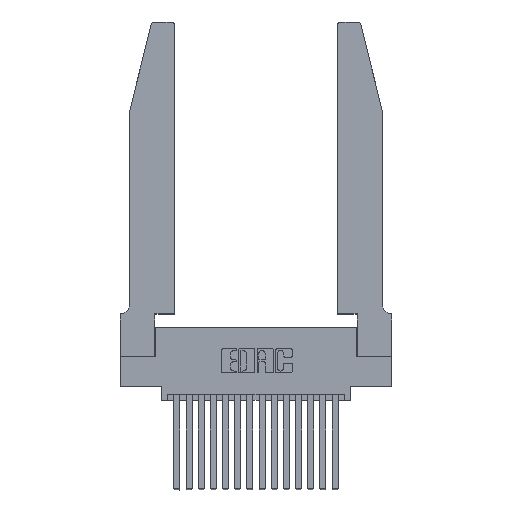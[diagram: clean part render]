
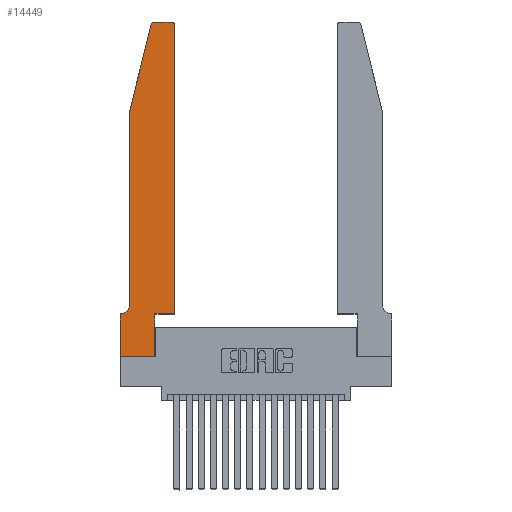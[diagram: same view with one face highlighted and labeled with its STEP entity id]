
A CAD part, top view. The second image highlights one B-rep face of the part: STEP entity #14449.
In plain terms, the highlighted planar face has unit normal (0, 0, 1).
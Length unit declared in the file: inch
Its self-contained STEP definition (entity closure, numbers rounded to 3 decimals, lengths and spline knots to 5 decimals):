
#177 = ORIENTED_EDGE ( 'NONE', *, *, #8714, .T. ) ;
#188 = AXIS2_PLACEMENT_3D ( 'NONE', #12216, #245, #10755 ) ;
#245 = DIRECTION ( 'NONE',  ( 0., 0., 1. ) ) ;
#603 = VERTEX_POINT ( 'NONE', #993 ) ;
#736 = VECTOR ( 'NONE', #13074, 39.37008 ) ;
#993 = CARTESIAN_POINT ( 'NONE',  ( 0.4505, 2.72, 0.37 ) ) ;
#1375 = AXIS2_PLACEMENT_3D ( 'NONE', #16887, #15448, #7917 ) ;
#1655 = AXIS2_PLACEMENT_3D ( 'NONE', #14983, #9304, #18419 ) ;
#1835 = EDGE_CURVE ( 'NONE', #2698, #10015, #9314, .T. ) ;
#1875 = LINE ( 'NONE', #9151, #5435 ) ;
#2230 = VERTEX_POINT ( 'NONE', #5632 ) ;
#2486 = DIRECTION ( 'NONE',  ( 0., 1., 0. ) ) ;
#2698 = VERTEX_POINT ( 'NONE', #7965 ) ;
#2702 = ORIENTED_EDGE ( 'NONE', *, *, #19317, .T. ) ;
#2794 = CARTESIAN_POINT ( 'NONE',  ( 0.0055, 0.42, 0.37 ) ) ;
#2867 = VECTOR ( 'NONE', #10861, 39.37008 ) ;
#2939 = DIRECTION ( 'NONE',  ( -0.239, -0.971, 0. ) ) ;
#3143 = CARTESIAN_POINT ( 'NONE',  ( 0.2865, 0.35, 0.37 ) ) ;
#3212 = EDGE_CURVE ( 'NONE', #603, #6087, #18404, .T. ) ;
#3765 = ORIENTED_EDGE ( 'NONE', *, *, #10191, .T. ) ;
#3843 = LINE ( 'NONE', #14655, #18168 ) ;
#3904 = ORIENTED_EDGE ( 'NONE', *, *, #5916, .T. ) ;
#4519 = LINE ( 'NONE', #13797, #14395 ) ;
#4533 = DIRECTION ( 'NONE',  ( 0., -1., 0. ) ) ;
#4868 = EDGE_CURVE ( 'NONE', #6087, #14637, #15301, .T. ) ;
#4906 = PLANE ( 'NONE',  #188 ) ;
#5160 = ORIENTED_EDGE ( 'NONE', *, *, #3212, .T. ) ;
#5254 = EDGE_CURVE ( 'NONE', #10039, #19252, #15999, .T. ) ;
#5353 = VECTOR ( 'NONE', #2939, 39.37008 ) ;
#5435 = VECTOR ( 'NONE', #12134, 39.37008 ) ;
#5632 = CARTESIAN_POINT ( 'NONE',  ( 0., 0., 0.37 ) ) ;
#5649 = EDGE_CURVE ( 'NONE', #10015, #10039, #1875, .T. ) ;
#5655 = ORIENTED_EDGE ( 'NONE', *, *, #5254, .T. ) ;
#5840 = EDGE_CURVE ( 'NONE', #2230, #12924, #9612, .T. ) ;
#5916 = EDGE_CURVE ( 'NONE', #12924, #14421, #11036, .T. ) ;
#5948 = CARTESIAN_POINT ( 'NONE',  ( 0.0755, 2., 0.37 ) ) ;
#6087 = VERTEX_POINT ( 'NONE', #14029 ) ;
#6096 = CARTESIAN_POINT ( 'NONE',  ( 0.4505, 0.35, 0.37 ) ) ;
#6678 = VECTOR ( 'NONE', #12892, 39.37008 ) ;
#7103 = ORIENTED_EDGE ( 'NONE', *, *, #1835, .T. ) ;
#7500 = ORIENTED_EDGE ( 'NONE', *, *, #4868, .T. ) ;
#7827 = FACE_OUTER_BOUND ( 'NONE', #16770, .T. ) ;
#7872 = LINE ( 'NONE', #15895, #6678 ) ;
#7917 = DIRECTION ( 'NONE',  ( 1., 0., 0. ) ) ;
#7965 = CARTESIAN_POINT ( 'NONE',  ( 0.25487, 2.72718, 0.37 ) ) ;
#8046 = CARTESIAN_POINT ( 'NONE',  ( 0.0055, 0.35, 0.37 ) ) ;
#8487 = CARTESIAN_POINT ( 'NONE',  ( 0.2865, 0., 0.37 ) ) ;
#8714 = EDGE_CURVE ( 'NONE', #19252, #11439, #7872, .T. ) ;
#8892 = DIRECTION ( 'NONE',  ( 0., 0., -1. ) ) ;
#9151 = CARTESIAN_POINT ( 'NONE',  ( 0.0755, 2., 0.37 ) ) ;
#9304 = DIRECTION ( 'NONE',  ( 0., 0., 1. ) ) ;
#9314 = LINE ( 'NONE', #11943, #5353 ) ;
#9600 = ORIENTED_EDGE ( 'NONE', *, *, #14201, .T. ) ;
#9612 = LINE ( 'NONE', #15589, #18309 ) ;
#9696 = VERTEX_POINT ( 'NONE', #13891 ) ;
#10015 = VERTEX_POINT ( 'NONE', #5948 ) ;
#10039 = VERTEX_POINT ( 'NONE', #10529 ) ;
#10191 = EDGE_CURVE ( 'NONE', #14421, #9696, #4519, .T. ) ;
#10529 = CARTESIAN_POINT ( 'NONE',  ( 0.0755, 0.42, 0.37 ) ) ;
#10755 = DIRECTION ( 'NONE',  ( 1., 0., 0. ) ) ;
#10861 = DIRECTION ( 'NONE',  ( 0., 1., 0. ) ) ;
#11036 = LINE ( 'NONE', #17312, #17366 ) ;
#11439 = VERTEX_POINT ( 'NONE', #15285 ) ;
#11865 = ORIENTED_EDGE ( 'NONE', *, *, #5649, .T. ) ;
#11943 = CARTESIAN_POINT ( 'NONE',  ( 0.0755, 2., 0.37 ) ) ;
#12134 = DIRECTION ( 'NONE',  ( 0., -1., 0. ) ) ;
#12172 = DIRECTION ( 'NONE',  ( 1., 0., 0. ) ) ;
#12216 = CARTESIAN_POINT ( 'NONE',  ( 0., 0.35, 0.37 ) ) ;
#12892 = DIRECTION ( 'NONE',  ( -1., 0., 0. ) ) ;
#12924 = VERTEX_POINT ( 'NONE', #8487 ) ;
#13074 = DIRECTION ( 'NONE',  ( -1., 0., 0. ) ) ;
#13797 = CARTESIAN_POINT ( 'NONE',  ( 0.4505, 0.35, 0.37 ) ) ;
#13891 = CARTESIAN_POINT ( 'NONE',  ( 0.4505, 0.35, 0.37 ) ) ;
#14029 = CARTESIAN_POINT ( 'NONE',  ( 0.4205, 2.75, 0.37 ) ) ;
#14201 = EDGE_CURVE ( 'NONE', #11439, #2230, #3843, .T. ) ;
#14395 = VECTOR ( 'NONE', #12172, 39.37008 ) ;
#14421 = VERTEX_POINT ( 'NONE', #3143 ) ;
#14449 = ADVANCED_FACE ( 'NONE', ( #7827 ), #4906, .T. ) ;
#14637 = VERTEX_POINT ( 'NONE', #15868 ) ;
#14655 = CARTESIAN_POINT ( 'NONE',  ( 0., 0., 0.37 ) ) ;
#14983 = CARTESIAN_POINT ( 'NONE',  ( 0.4205, 2.72, 0.37 ) ) ;
#15040 = EDGE_CURVE ( 'NONE', #9696, #603, #15531, .T. ) ;
#15237 = ORIENTED_EDGE ( 'NONE', *, *, #15040, .T. ) ;
#15285 = CARTESIAN_POINT ( 'NONE',  ( 0., 0.35, 0.37 ) ) ;
#15301 = LINE ( 'NONE', #17565, #736 ) ;
#15448 = DIRECTION ( 'NONE',  ( 0., 0., 1. ) ) ;
#15531 = LINE ( 'NONE', #6096, #2867 ) ;
#15589 = CARTESIAN_POINT ( 'NONE',  ( 0., 0., 0.37 ) ) ;
#15868 = CARTESIAN_POINT ( 'NONE',  ( 0.284, 2.75, 0.37 ) ) ;
#15895 = CARTESIAN_POINT ( 'NONE',  ( 0.0755, 0.35, 0.37 ) ) ;
#15999 = CIRCLE ( 'NONE', #16894, 0.07 ) ;
#16246 = DIRECTION ( 'NONE',  ( -1., 0., 0. ) ) ;
#16770 = EDGE_LOOP ( 'NONE', ( #7500, #2702, #7103, #11865, #5655, #177, #9600, #18312, #3904, #3765, #15237, #5160 ) ) ;
#16887 = CARTESIAN_POINT ( 'NONE',  ( 0.284, 2.72, 0.37 ) ) ;
#16894 = AXIS2_PLACEMENT_3D ( 'NONE', #2794, #8892, #16246 ) ;
#17081 = DIRECTION ( 'NONE',  ( 1., 0., 0. ) ) ;
#17312 = CARTESIAN_POINT ( 'NONE',  ( 0.2865, 0.35, 0.37 ) ) ;
#17366 = VECTOR ( 'NONE', #2486, 39.37008 ) ;
#17458 = CIRCLE ( 'NONE', #1375, 0.03 ) ;
#17565 = CARTESIAN_POINT ( 'NONE',  ( 0.2605, 2.75, 0.37 ) ) ;
#18168 = VECTOR ( 'NONE', #4533, 39.37008 ) ;
#18309 = VECTOR ( 'NONE', #17081, 39.37008 ) ;
#18312 = ORIENTED_EDGE ( 'NONE', *, *, #5840, .T. ) ;
#18404 = CIRCLE ( 'NONE', #1655, 0.03 ) ;
#18419 = DIRECTION ( 'NONE',  ( 1., 0., 0. ) ) ;
#19252 = VERTEX_POINT ( 'NONE', #8046 ) ;
#19317 = EDGE_CURVE ( 'NONE', #14637, #2698, #17458, .T. ) ;
